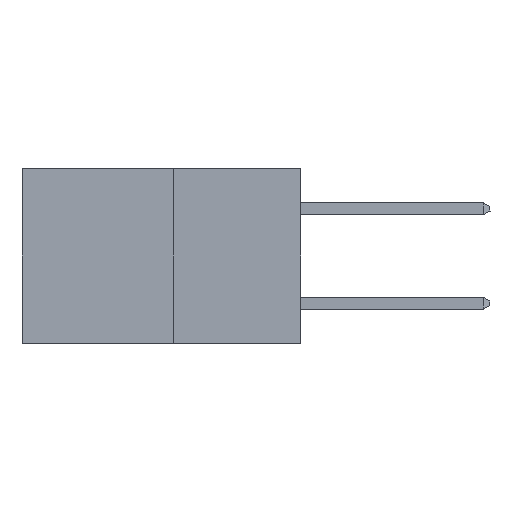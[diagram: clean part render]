
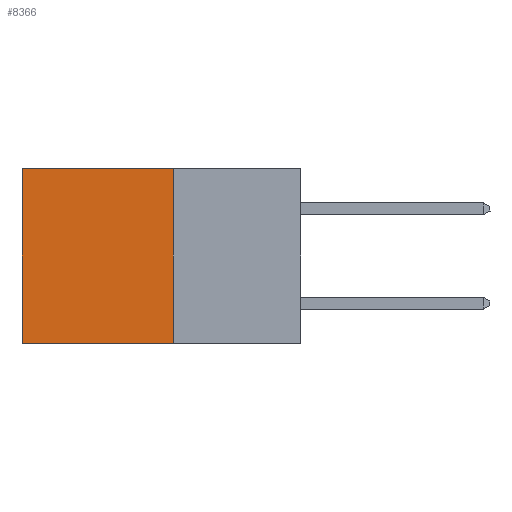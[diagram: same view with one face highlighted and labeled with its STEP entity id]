
A CAD part, left-side view. The second image highlights one B-rep face of the part: STEP entity #8366.
In plain terms, the highlighted planar face has unit normal (-1, 0, 0).
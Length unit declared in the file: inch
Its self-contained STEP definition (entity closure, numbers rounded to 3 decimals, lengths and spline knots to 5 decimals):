
#1772 = VECTOR ( 'NONE', #15635, 39.37008 ) ;
#2642 = EDGE_LOOP ( 'NONE', ( #12080, #12404, #14226, #13727 ) ) ;
#3219 = DIRECTION ( 'NONE',  ( 0., 1., 0. ) ) ;
#3347 = CARTESIAN_POINT ( 'NONE',  ( 0.277, 0.27, 0. ) ) ;
#4836 = EDGE_CURVE ( 'NONE', #11899, #11522, #11974, .T. ) ;
#5012 = LINE ( 'NONE', #13876, #12301 ) ;
#5163 = DIRECTION ( 'NONE',  ( 0., 1., 0. ) ) ;
#6194 = VERTEX_POINT ( 'NONE', #7442 ) ;
#7338 = CARTESIAN_POINT ( 'NONE',  ( 0.277, 0.27, -0.37 ) ) ;
#7442 = CARTESIAN_POINT ( 'NONE',  ( 0.277, 0.27, 0. ) ) ;
#7751 = DIRECTION ( 'NONE',  ( 0., 0., -1. ) ) ;
#7807 = VERTEX_POINT ( 'NONE', #7338 ) ;
#8024 = CARTESIAN_POINT ( 'NONE',  ( 0.277, 0.59, -0.37 ) ) ;
#8366 = ADVANCED_FACE ( 'NONE', ( #13457 ), #16743, .F. ) ;
#8411 = DIRECTION ( 'NONE',  ( 0., 0., -1. ) ) ;
#9113 = EDGE_CURVE ( 'NONE', #7807, #11522, #5012, .T. ) ;
#9591 = LINE ( 'NONE', #15671, #1772 ) ;
#10590 = CARTESIAN_POINT ( 'NONE',  ( 0.277, 0.59, -0.37 ) ) ;
#10723 = VECTOR ( 'NONE', #3219, 39.37008 ) ;
#10849 = CARTESIAN_POINT ( 'NONE',  ( 0.277, 0.59, 0. ) ) ;
#11176 = LINE ( 'NONE', #3347, #10723 ) ;
#11522 = VERTEX_POINT ( 'NONE', #10590 ) ;
#11899 = VERTEX_POINT ( 'NONE', #10849 ) ;
#11974 = LINE ( 'NONE', #8024, #12443 ) ;
#12080 = ORIENTED_EDGE ( 'NONE', *, *, #4836, .T. ) ;
#12301 = VECTOR ( 'NONE', #5163, 39.37008 ) ;
#12404 = ORIENTED_EDGE ( 'NONE', *, *, #9113, .F. ) ;
#12443 = VECTOR ( 'NONE', #7751, 39.37008 ) ;
#13457 = FACE_OUTER_BOUND ( 'NONE', #2642, .T. ) ;
#13567 = AXIS2_PLACEMENT_3D ( 'NONE', #17682, #15881, #8411 ) ;
#13727 = ORIENTED_EDGE ( 'NONE', *, *, #17770, .T. ) ;
#13871 = EDGE_CURVE ( 'NONE', #6194, #7807, #9591, .T. ) ;
#13876 = CARTESIAN_POINT ( 'NONE',  ( 0.277, 0.27, -0.37 ) ) ;
#14226 = ORIENTED_EDGE ( 'NONE', *, *, #13871, .F. ) ;
#15635 = DIRECTION ( 'NONE',  ( 0., 0., -1. ) ) ;
#15671 = CARTESIAN_POINT ( 'NONE',  ( 0.277, 0.27, -0.37 ) ) ;
#15881 = DIRECTION ( 'NONE',  ( 1., 0., 0. ) ) ;
#16743 = PLANE ( 'NONE',  #13567 ) ;
#17682 = CARTESIAN_POINT ( 'NONE',  ( 0.277, 0.27, -0.37 ) ) ;
#17770 = EDGE_CURVE ( 'NONE', #6194, #11899, #11176, .T. ) ;
